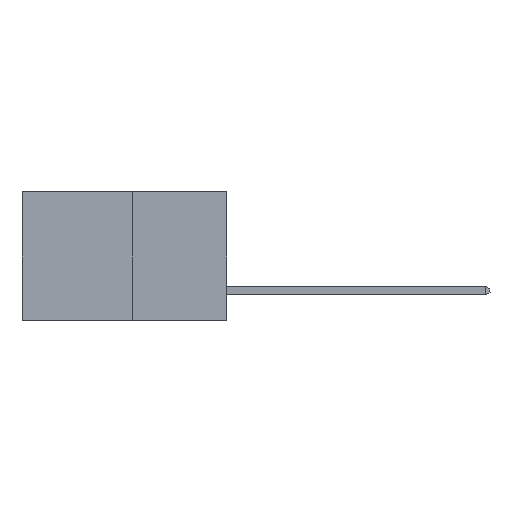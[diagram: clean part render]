
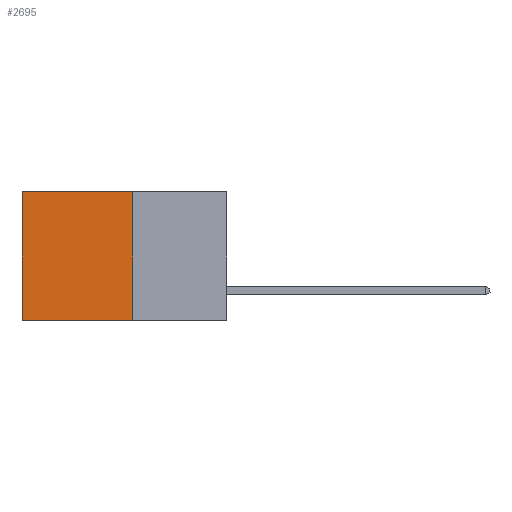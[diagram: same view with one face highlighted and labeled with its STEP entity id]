
A CAD part, left-side view. The second image highlights one B-rep face of the part: STEP entity #2695.
In plain terms, the highlighted planar face has unit normal (-1, 0, 0).
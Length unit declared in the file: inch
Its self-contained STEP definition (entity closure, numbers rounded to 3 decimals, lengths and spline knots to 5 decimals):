
#661 = VECTOR ( 'NONE', #9898, 39.37008 ) ;
#853 = ORIENTED_EDGE ( 'NONE', *, *, #10703, .F. ) ;
#889 = CARTESIAN_POINT ( 'NONE',  ( 0.277, 0.59, 0. ) ) ;
#1107 = VERTEX_POINT ( 'NONE', #889 ) ;
#1267 = VERTEX_POINT ( 'NONE', #12057 ) ;
#1730 = CARTESIAN_POINT ( 'NONE',  ( 0.277, 0.27, -0.37 ) ) ;
#1983 = VECTOR ( 'NONE', #2902, 39.37008 ) ;
#2695 = ADVANCED_FACE ( 'NONE', ( #4558 ), #6258, .F. ) ;
#2902 = DIRECTION ( 'NONE',  ( 0., 0., -1. ) ) ;
#2950 = DIRECTION ( 'NONE',  ( 0., 1., 0. ) ) ;
#3795 = LINE ( 'NONE', #10070, #661 ) ;
#3897 = CARTESIAN_POINT ( 'NONE',  ( 0.277, 0.27, -0.37 ) ) ;
#4558 = FACE_OUTER_BOUND ( 'NONE', #7554, .T. ) ;
#5046 = LINE ( 'NONE', #1730, #1983 ) ;
#5047 = EDGE_CURVE ( 'NONE', #1107, #1267, #3795, .T. ) ;
#5900 = VERTEX_POINT ( 'NONE', #3897 ) ;
#6073 = LINE ( 'NONE', #11452, #11632 ) ;
#6258 = PLANE ( 'NONE',  #7869 ) ;
#6419 = EDGE_CURVE ( 'NONE', #7033, #1107, #6073, .T. ) ;
#7033 = VERTEX_POINT ( 'NONE', #9226 ) ;
#7554 = EDGE_LOOP ( 'NONE', ( #8251, #10898, #853, #13388 ) ) ;
#7618 = EDGE_CURVE ( 'NONE', #5900, #1267, #12604, .T. ) ;
#7869 = AXIS2_PLACEMENT_3D ( 'NONE', #12261, #12258, #11806 ) ;
#8251 = ORIENTED_EDGE ( 'NONE', *, *, #5047, .T. ) ;
#9226 = CARTESIAN_POINT ( 'NONE',  ( 0.277, 0.27, 0. ) ) ;
#9684 = CARTESIAN_POINT ( 'NONE',  ( 0.277, 0.27, -0.37 ) ) ;
#9898 = DIRECTION ( 'NONE',  ( 0., 0., -1. ) ) ;
#10070 = CARTESIAN_POINT ( 'NONE',  ( 0.277, 0.59, -0.37 ) ) ;
#10703 = EDGE_CURVE ( 'NONE', #7033, #5900, #5046, .T. ) ;
#10898 = ORIENTED_EDGE ( 'NONE', *, *, #7618, .F. ) ;
#11304 = DIRECTION ( 'NONE',  ( 0., 1., 0. ) ) ;
#11452 = CARTESIAN_POINT ( 'NONE',  ( 0.277, 0.27, 0. ) ) ;
#11632 = VECTOR ( 'NONE', #11304, 39.37008 ) ;
#11806 = DIRECTION ( 'NONE',  ( 0., 0., -1. ) ) ;
#12057 = CARTESIAN_POINT ( 'NONE',  ( 0.277, 0.59, -0.37 ) ) ;
#12258 = DIRECTION ( 'NONE',  ( 1., 0., 0. ) ) ;
#12261 = CARTESIAN_POINT ( 'NONE',  ( 0.277, 0.27, -0.37 ) ) ;
#12604 = LINE ( 'NONE', #9684, #12954 ) ;
#12954 = VECTOR ( 'NONE', #2950, 39.37008 ) ;
#13388 = ORIENTED_EDGE ( 'NONE', *, *, #6419, .T. ) ;
